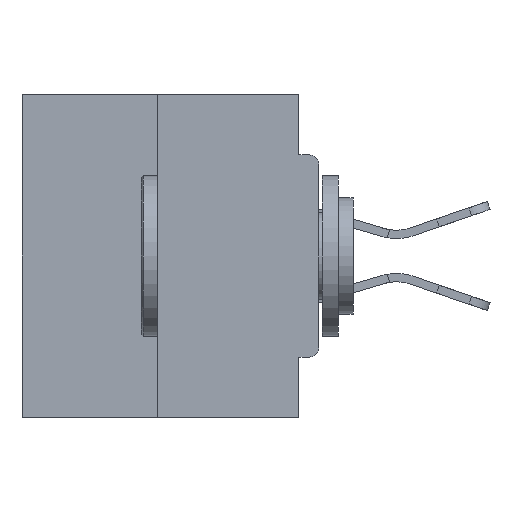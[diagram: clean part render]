
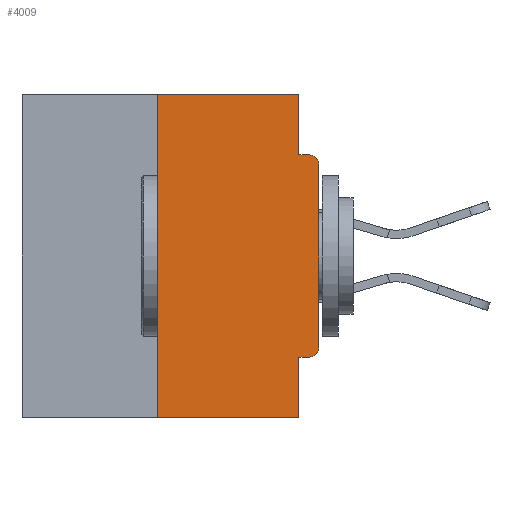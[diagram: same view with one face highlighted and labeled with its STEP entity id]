
A CAD part, left-side view. The second image highlights one B-rep face of the part: STEP entity #4009.
In plain terms, the highlighted planar face has unit normal (-1, 0, 0).
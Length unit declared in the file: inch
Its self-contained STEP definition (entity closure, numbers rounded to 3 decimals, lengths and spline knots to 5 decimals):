
#781 = CIRCLE ( 'NONE', #23460, 0.015 ) ;
#1572 = EDGE_CURVE ( 'NONE', #13251, #6969, #10629, .T. ) ;
#1753 = DIRECTION ( 'NONE',  ( 0., 0., -1. ) ) ;
#2055 = VERTEX_POINT ( 'NONE', #29103 ) ;
#3337 = VECTOR ( 'NONE', #3521, 39.37008 ) ;
#3521 = DIRECTION ( 'NONE',  ( 0., -1., 0. ) ) ;
#3575 = VERTEX_POINT ( 'NONE', #7289 ) ;
#3637 = CARTESIAN_POINT ( 'NONE',  ( 0., 0., -0.0935 ) ) ;
#3744 = CARTESIAN_POINT ( 'NONE',  ( 0., 0.031, -0.4065 ) ) ;
#4009 = ADVANCED_FACE ( 'NONE', ( #9178 ), #23513, .F. ) ;
#4248 = VECTOR ( 'NONE', #31487, 39.37008 ) ;
#4676 = LINE ( 'NONE', #9609, #4248 ) ;
#5161 = CARTESIAN_POINT ( 'NONE',  ( 0., 0.015, -0.4065 ) ) ;
#5431 = VECTOR ( 'NONE', #26507, 39.37008 ) ;
#5659 = ORIENTED_EDGE ( 'NONE', *, *, #1572, .F. ) ;
#6192 = EDGE_CURVE ( 'NONE', #27177, #13251, #4676, .T. ) ;
#6365 = DIRECTION ( 'NONE',  ( 0., 1., 0. ) ) ;
#6948 = VERTEX_POINT ( 'NONE', #33983 ) ;
#6969 = VERTEX_POINT ( 'NONE', #23187 ) ;
#7289 = CARTESIAN_POINT ( 'NONE',  ( 0., 0., -0.1085 ) ) ;
#7987 = VECTOR ( 'NONE', #26031, 39.37008 ) ;
#8074 = EDGE_CURVE ( 'NONE', #24331, #2055, #20049, .T. ) ;
#8364 = EDGE_CURVE ( 'NONE', #13951, #6948, #33394, .T. ) ;
#8735 = CARTESIAN_POINT ( 'NONE',  ( 0., 0., -0.4065 ) ) ;
#9142 = CARTESIAN_POINT ( 'NONE',  ( 0., 0.015, -0.1085 ) ) ;
#9178 = FACE_OUTER_BOUND ( 'NONE', #29314, .T. ) ;
#9325 = VECTOR ( 'NONE', #6365, 39.37008 ) ;
#9609 = CARTESIAN_POINT ( 'NONE',  ( 0., 0.031, 0. ) ) ;
#10002 = AXIS2_PLACEMENT_3D ( 'NONE', #28877, #12551, #1753 ) ;
#10629 = LINE ( 'NONE', #3637, #3337 ) ;
#11189 = ORIENTED_EDGE ( 'NONE', *, *, #8364, .T. ) ;
#12051 = DIRECTION ( 'NONE',  ( -1., 0., 0. ) ) ;
#12177 = ORIENTED_EDGE ( 'NONE', *, *, #6192, .F. ) ;
#12216 = VECTOR ( 'NONE', #18688, 39.37008 ) ;
#12457 = EDGE_CURVE ( 'NONE', #3575, #6969, #781, .T. ) ;
#12551 = DIRECTION ( 'NONE',  ( -1., 0., 0. ) ) ;
#13042 = LINE ( 'NONE', #24323, #12216 ) ;
#13251 = VERTEX_POINT ( 'NONE', #28858 ) ;
#13573 = CARTESIAN_POINT ( 'NONE',  ( 0., 0.25, 0. ) ) ;
#13951 = VERTEX_POINT ( 'NONE', #19535 ) ;
#14108 = EDGE_CURVE ( 'NONE', #28056, #6948, #34018, .T. ) ;
#14672 = DIRECTION ( 'NONE',  ( 0., -1., 0. ) ) ;
#14992 = DIRECTION ( 'NONE',  ( 1., 0., 0. ) ) ;
#15620 = CARTESIAN_POINT ( 'NONE',  ( 0., 0.031, 0. ) ) ;
#16065 = EDGE_CURVE ( 'NONE', #2055, #3575, #35551, .T. ) ;
#18688 = DIRECTION ( 'NONE',  ( 0., 0., 1. ) ) ;
#19535 = CARTESIAN_POINT ( 'NONE',  ( 0., 0.25, -0.5 ) ) ;
#19890 = LINE ( 'NONE', #20620, #35398 ) ;
#19963 = DIRECTION ( 'NONE',  ( 0., 0., -1. ) ) ;
#20018 = CARTESIAN_POINT ( 'NONE',  ( 0., 0.031, -0.5 ) ) ;
#20049 = CIRCLE ( 'NONE', #10002, 0.015 ) ;
#20620 = CARTESIAN_POINT ( 'NONE',  ( 0., 0.46, 0. ) ) ;
#21957 = VERTEX_POINT ( 'NONE', #13573 ) ;
#22405 = EDGE_CURVE ( 'NONE', #13951, #21957, #13042, .T. ) ;
#22506 = DIRECTION ( 'NONE',  ( 0., 0., -1. ) ) ;
#22641 = LINE ( 'NONE', #8735, #9325 ) ;
#23187 = CARTESIAN_POINT ( 'NONE',  ( 0., 0.015, -0.0935 ) ) ;
#23262 = CARTESIAN_POINT ( 'NONE',  ( 0., 0., 0. ) ) ;
#23277 = DIRECTION ( 'NONE',  ( 0., 0., -1. ) ) ;
#23460 = AXIS2_PLACEMENT_3D ( 'NONE', #9142, #12051, #19963 ) ;
#23513 = PLANE ( 'NONE',  #27299 ) ;
#24323 = CARTESIAN_POINT ( 'NONE',  ( 0., 0.25, 0. ) ) ;
#24331 = VERTEX_POINT ( 'NONE', #5161 ) ;
#25392 = ORIENTED_EDGE ( 'NONE', *, *, #35003, .F. ) ;
#25589 = CARTESIAN_POINT ( 'NONE',  ( 0., 0.46, -0.5 ) ) ;
#26031 = DIRECTION ( 'NONE',  ( 0., 0., 1. ) ) ;
#26507 = DIRECTION ( 'NONE',  ( 0., -1., 0. ) ) ;
#27177 = VERTEX_POINT ( 'NONE', #15620 ) ;
#27299 = AXIS2_PLACEMENT_3D ( 'NONE', #34177, #14992, #23277 ) ;
#28056 = VERTEX_POINT ( 'NONE', #3744 ) ;
#28858 = CARTESIAN_POINT ( 'NONE',  ( 0., 0.031, -0.0935 ) ) ;
#28877 = CARTESIAN_POINT ( 'NONE',  ( 0., 0.015, -0.3915 ) ) ;
#29103 = CARTESIAN_POINT ( 'NONE',  ( 0., 0., -0.3915 ) ) ;
#29314 = EDGE_LOOP ( 'NONE', ( #29677, #29545, #11189, #29831, #25392, #34752, #30868, #29737, #5659, #12177 ) ) ;
#29545 = ORIENTED_EDGE ( 'NONE', *, *, #22405, .F. ) ;
#29677 = ORIENTED_EDGE ( 'NONE', *, *, #33369, .F. ) ;
#29737 = ORIENTED_EDGE ( 'NONE', *, *, #12457, .T. ) ;
#29831 = ORIENTED_EDGE ( 'NONE', *, *, #14108, .F. ) ;
#30868 = ORIENTED_EDGE ( 'NONE', *, *, #16065, .T. ) ;
#31487 = DIRECTION ( 'NONE',  ( 0., 0., -1. ) ) ;
#33129 = VECTOR ( 'NONE', #22506, 39.37008 ) ;
#33369 = EDGE_CURVE ( 'NONE', #21957, #27177, #19890, .T. ) ;
#33394 = LINE ( 'NONE', #25589, #5431 ) ;
#33983 = CARTESIAN_POINT ( 'NONE',  ( 0., 0.031, -0.5 ) ) ;
#34018 = LINE ( 'NONE', #20018, #33129 ) ;
#34177 = CARTESIAN_POINT ( 'NONE',  ( 0., 0.46, 0. ) ) ;
#34752 = ORIENTED_EDGE ( 'NONE', *, *, #8074, .T. ) ;
#35003 = EDGE_CURVE ( 'NONE', #24331, #28056, #22641, .T. ) ;
#35398 = VECTOR ( 'NONE', #14672, 39.37008 ) ;
#35551 = LINE ( 'NONE', #23262, #7987 ) ;
